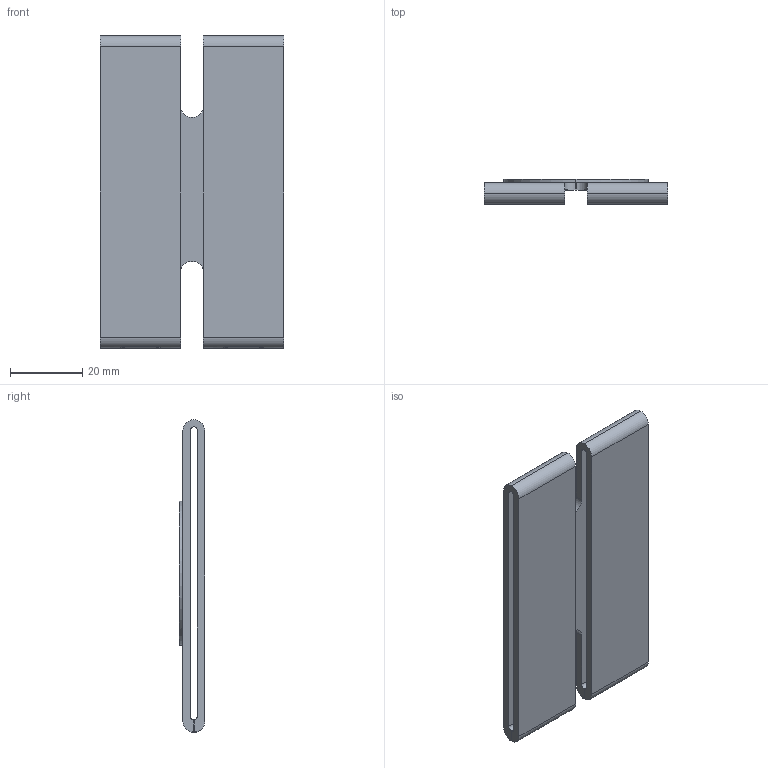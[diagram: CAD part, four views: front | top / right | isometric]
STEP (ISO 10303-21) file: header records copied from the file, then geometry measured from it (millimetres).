
FILE_DESCRIPTION (( 'STEP AP214' ), '1' );
FILE_NAME ('Molle Clip.STEP', '2013-07-17T19:15:37', ( 'Asher' ), ( '' ), 'SwSTEP 2.0', 'SolidWorks 2013', '' );
FILE_SCHEMA (( 'AUTOMOTIVE_DESIGN' ));
Length unit declared in the file: millimetre
Products named in the file (1): Molle Clip
Bounding box: 50.8 x 7 x 86.74 mm (x, y, z)
Volume: 17356.3 mm3; surface area: 17559.4 mm2
Topology: 1 solids, 1 shells, 137 faces, 369 edges, 226 vertices
Faces by surface type: cylinder 73, plane 32, bspline 32
Entity records: 5175 total; most frequent: CARTESIAN_POINT 2071, ORIENTED_EDGE 722, DIRECTION 559, EDGE_CURVE 361, VERTEX_POINT 226, AXIS2_PLACEMENT_3D 206, VECTOR 147, LINE 147
